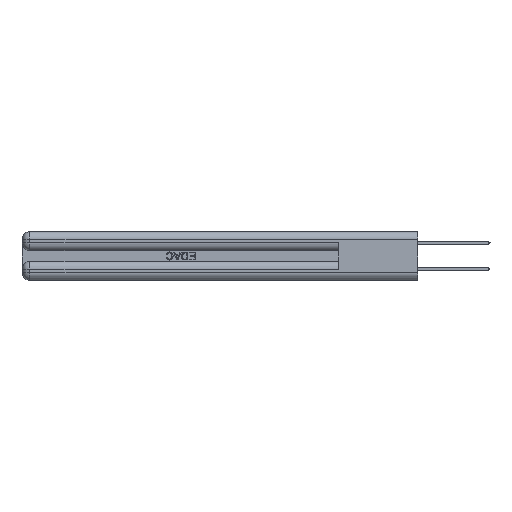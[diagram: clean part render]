
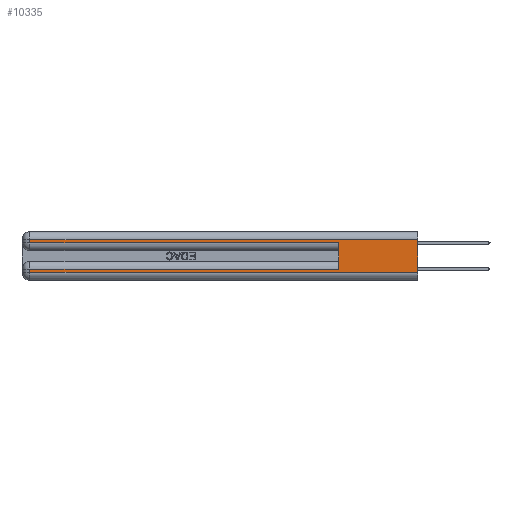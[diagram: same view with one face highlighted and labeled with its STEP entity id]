
A CAD part, left-side view. The second image highlights one B-rep face of the part: STEP entity #10335.
In plain terms, the highlighted planar face has unit normal (-1, 0, 0).
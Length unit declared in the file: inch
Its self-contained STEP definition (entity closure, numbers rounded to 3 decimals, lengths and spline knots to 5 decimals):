
#420 = DIRECTION ( 'NONE',  ( 0., 0., -1. ) ) ;
#908 = EDGE_CURVE ( 'NONE', #18361, #45067, #43725, .T. ) ;
#1230 = DIRECTION ( 'NONE',  ( 0., -1., 0. ) ) ;
#2649 = VECTOR ( 'NONE', #11066, 39.37008 ) ;
#3298 = DIRECTION ( 'NONE',  ( 0., 0., -1. ) ) ;
#3741 = CARTESIAN_POINT ( 'NONE',  ( 0., 2.94, 0.37 ) ) ;
#3816 = VECTOR ( 'NONE', #10654, 39.37008 ) ;
#4009 = AXIS2_PLACEMENT_3D ( 'NONE', #4662, #40347, #36965 ) ;
#4283 = VECTOR ( 'NONE', #3298, 39.37008 ) ;
#4662 = CARTESIAN_POINT ( 'NONE',  ( 0., 0., 0.37 ) ) ;
#5061 = CARTESIAN_POINT ( 'NONE',  ( 0., 2.94, 0.06 ) ) ;
#5260 = ORIENTED_EDGE ( 'NONE', *, *, #31009, .T. ) ;
#6022 = LINE ( 'NONE', #17101, #3816 ) ;
#6496 = LINE ( 'NONE', #3741, #4283 ) ;
#8329 = ORIENTED_EDGE ( 'NONE', *, *, #35396, .F. ) ;
#9528 = EDGE_CURVE ( 'NONE', #21263, #42447, #18057, .T. ) ;
#10335 = ADVANCED_FACE ( 'NONE', ( #33905 ), #31425, .F. ) ;
#10654 = DIRECTION ( 'NONE',  ( 0., -1., 0. ) ) ;
#11053 = LINE ( 'NONE', #32897, #19271 ) ;
#11066 = DIRECTION ( 'NONE',  ( 0., 1., 0. ) ) ;
#11857 = VERTEX_POINT ( 'NONE', #26953 ) ;
#13720 = CARTESIAN_POINT ( 'NONE',  ( 0., 2.94, 0.31 ) ) ;
#13873 = EDGE_CURVE ( 'NONE', #27950, #21263, #33021, .T. ) ;
#17101 = CARTESIAN_POINT ( 'NONE',  ( 0., 0., 0.06 ) ) ;
#18057 = LINE ( 'NONE', #37685, #21344 ) ;
#18361 = VERTEX_POINT ( 'NONE', #30574 ) ;
#18574 = DIRECTION ( 'NONE',  ( 0., 0., 1. ) ) ;
#19271 = VECTOR ( 'NONE', #1230, 39.37008 ) ;
#21263 = VERTEX_POINT ( 'NONE', #36482 ) ;
#21344 = VECTOR ( 'NONE', #27239, 39.37008 ) ;
#21378 = ORIENTED_EDGE ( 'NONE', *, *, #9528, .T. ) ;
#22656 = ORIENTED_EDGE ( 'NONE', *, *, #31648, .F. ) ;
#25326 = CARTESIAN_POINT ( 'NONE',  ( 0., 0.6, 0.085 ) ) ;
#25742 = EDGE_CURVE ( 'NONE', #42447, #33460, #6022, .T. ) ;
#25826 = VECTOR ( 'NONE', #18574, 39.37008 ) ;
#26866 = CARTESIAN_POINT ( 'NONE',  ( 0., 2.94, 0.285 ) ) ;
#26953 = CARTESIAN_POINT ( 'NONE',  ( 0., 0.6, 0.285 ) ) ;
#27239 = DIRECTION ( 'NONE',  ( 0., 0., -1. ) ) ;
#27950 = VERTEX_POINT ( 'NONE', #25326 ) ;
#28151 = CARTESIAN_POINT ( 'NONE',  ( 0., 0., 0.06 ) ) ;
#29791 = ORIENTED_EDGE ( 'NONE', *, *, #25742, .T. ) ;
#29989 = ORIENTED_EDGE ( 'NONE', *, *, #908, .T. ) ;
#30574 = CARTESIAN_POINT ( 'NONE',  ( 0., 0., 0.31 ) ) ;
#30862 = VECTOR ( 'NONE', #33725, 39.37008 ) ;
#31009 = EDGE_CURVE ( 'NONE', #45067, #41560, #6496, .T. ) ;
#31425 = PLANE ( 'NONE',  #4009 ) ;
#31648 = EDGE_CURVE ( 'NONE', #18361, #33460, #37643, .T. ) ;
#32897 = CARTESIAN_POINT ( 'NONE',  ( 0., 0., 0.285 ) ) ;
#33021 = LINE ( 'NONE', #44184, #30862 ) ;
#33460 = VERTEX_POINT ( 'NONE', #28151 ) ;
#33725 = DIRECTION ( 'NONE',  ( 0., 1., 0. ) ) ;
#33905 = FACE_OUTER_BOUND ( 'NONE', #44344, .T. ) ;
#34873 = VECTOR ( 'NONE', #420, 39.37008 ) ;
#35057 = ORIENTED_EDGE ( 'NONE', *, *, #13873, .T. ) ;
#35151 = LINE ( 'NONE', #42949, #25826 ) ;
#35396 = EDGE_CURVE ( 'NONE', #27950, #11857, #35151, .T. ) ;
#36482 = CARTESIAN_POINT ( 'NONE',  ( 0., 2.94, 0.085 ) ) ;
#36965 = DIRECTION ( 'NONE',  ( 0., 0., -1. ) ) ;
#37643 = LINE ( 'NONE', #42269, #34873 ) ;
#37685 = CARTESIAN_POINT ( 'NONE',  ( 0., 2.94, 0.37 ) ) ;
#40336 = ORIENTED_EDGE ( 'NONE', *, *, #41902, .T. ) ;
#40347 = DIRECTION ( 'NONE',  ( 1., 0., 0. ) ) ;
#41560 = VERTEX_POINT ( 'NONE', #26866 ) ;
#41869 = CARTESIAN_POINT ( 'NONE',  ( 0., 0., 0.31 ) ) ;
#41902 = EDGE_CURVE ( 'NONE', #41560, #11857, #11053, .T. ) ;
#42269 = CARTESIAN_POINT ( 'NONE',  ( 0., 0., 0.37 ) ) ;
#42447 = VERTEX_POINT ( 'NONE', #5061 ) ;
#42949 = CARTESIAN_POINT ( 'NONE',  ( 0., 0.6, 0.145 ) ) ;
#43725 = LINE ( 'NONE', #41869, #2649 ) ;
#44184 = CARTESIAN_POINT ( 'NONE',  ( 0., 0., 0.085 ) ) ;
#44344 = EDGE_LOOP ( 'NONE', ( #22656, #29989, #5260, #40336, #8329, #35057, #21378, #29791 ) ) ;
#45067 = VERTEX_POINT ( 'NONE', #13720 ) ;
